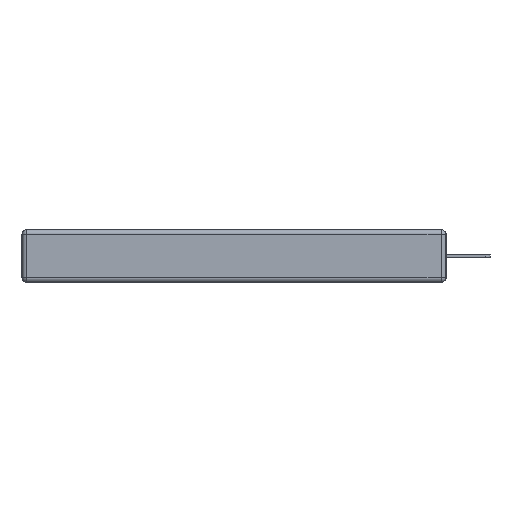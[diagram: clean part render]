
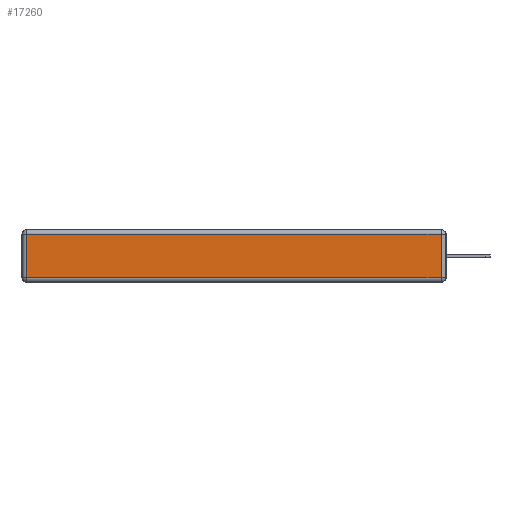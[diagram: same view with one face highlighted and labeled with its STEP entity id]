
A CAD part, left-side view. The second image highlights one B-rep face of the part: STEP entity #17260.
In plain terms, the highlighted planar face has unit normal (-1, 0, 0).
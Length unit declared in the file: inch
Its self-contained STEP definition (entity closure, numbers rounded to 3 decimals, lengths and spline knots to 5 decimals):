
#411 = AXIS2_PLACEMENT_3D ( 'NONE', #18012, #10362, #14806 ) ;
#1383 = EDGE_CURVE ( 'NONE', #10263, #8461, #8104, .T. ) ;
#1688 = DIRECTION ( 'NONE',  ( 0., 0., -1. ) ) ;
#3390 = CARTESIAN_POINT ( 'NONE',  ( 0., 2.75, -0.03 ) ) ;
#3777 = VERTEX_POINT ( 'NONE', #10526 ) ;
#3783 = ORIENTED_EDGE ( 'NONE', *, *, #8832, .T. ) ;
#4952 = ORIENTED_EDGE ( 'NONE', *, *, #18604, .T. ) ;
#5784 = ORIENTED_EDGE ( 'NONE', *, *, #1383, .T. ) ;
#6061 = DIRECTION ( 'NONE',  ( 0., 1., 0. ) ) ;
#6518 = VECTOR ( 'NONE', #6637, 39.37008 ) ;
#6637 = DIRECTION ( 'NONE',  ( 0., -1., 0. ) ) ;
#6965 = VECTOR ( 'NONE', #6061, 39.37008 ) ;
#6997 = VERTEX_POINT ( 'NONE', #17700 ) ;
#8104 = LINE ( 'NONE', #8200, #6518 ) ;
#8200 = CARTESIAN_POINT ( 'NONE',  ( 0., 0., -0.313 ) ) ;
#8461 = VERTEX_POINT ( 'NONE', #12726 ) ;
#8832 = EDGE_CURVE ( 'NONE', #8461, #3777, #17242, .T. ) ;
#9073 = EDGE_LOOP ( 'NONE', ( #5784, #3783, #11653, #4952 ) ) ;
#10263 = VERTEX_POINT ( 'NONE', #16109 ) ;
#10362 = DIRECTION ( 'NONE',  ( -1., 0., 0. ) ) ;
#10526 = CARTESIAN_POINT ( 'NONE',  ( 0., 0.03, -0.03 ) ) ;
#11653 = ORIENTED_EDGE ( 'NONE', *, *, #16731, .T. ) ;
#11997 = VECTOR ( 'NONE', #1688, 39.37008 ) ;
#12726 = CARTESIAN_POINT ( 'NONE',  ( 0., 0.03, -0.313 ) ) ;
#13946 = DIRECTION ( 'NONE',  ( 0., 0., 1. ) ) ;
#14191 = LINE ( 'NONE', #14590, #11997 ) ;
#14590 = CARTESIAN_POINT ( 'NONE',  ( 0., 2.72, -0.343 ) ) ;
#14806 = DIRECTION ( 'NONE',  ( 0., 0., 1. ) ) ;
#14905 = FACE_OUTER_BOUND ( 'NONE', #9073, .T. ) ;
#16109 = CARTESIAN_POINT ( 'NONE',  ( 0., 2.72, -0.313 ) ) ;
#16731 = EDGE_CURVE ( 'NONE', #3777, #6997, #17545, .T. ) ;
#17037 = CARTESIAN_POINT ( 'NONE',  ( 0., 0.03, -0.343 ) ) ;
#17242 = LINE ( 'NONE', #17037, #18449 ) ;
#17260 = ADVANCED_FACE ( 'NONE', ( #14905 ), #19364, .T. ) ;
#17545 = LINE ( 'NONE', #3390, #6965 ) ;
#17700 = CARTESIAN_POINT ( 'NONE',  ( 0., 2.72, -0.03 ) ) ;
#18012 = CARTESIAN_POINT ( 'NONE',  ( 0., 0., -0.343 ) ) ;
#18449 = VECTOR ( 'NONE', #13946, 39.37008 ) ;
#18604 = EDGE_CURVE ( 'NONE', #6997, #10263, #14191, .T. ) ;
#19364 = PLANE ( 'NONE',  #411 ) ;
